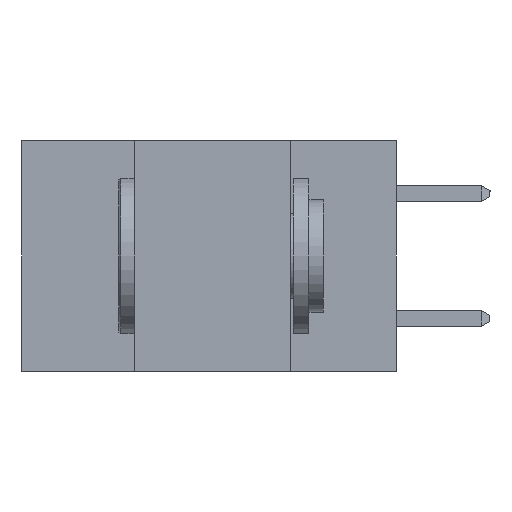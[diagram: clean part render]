
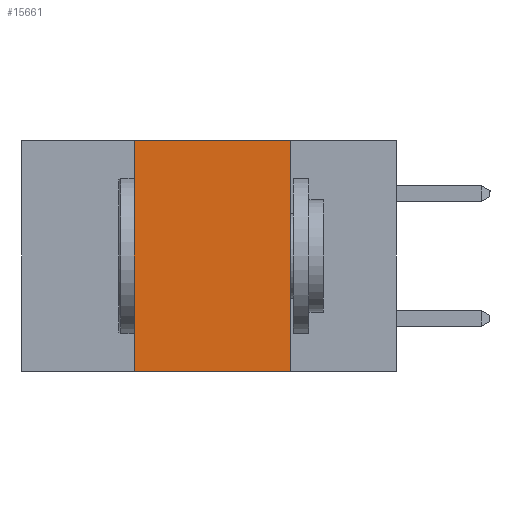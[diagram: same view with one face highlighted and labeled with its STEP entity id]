
A CAD part, left-side view. The second image highlights one B-rep face of the part: STEP entity #15661.
In plain terms, the highlighted planar face has unit normal (-1, 0, 0).
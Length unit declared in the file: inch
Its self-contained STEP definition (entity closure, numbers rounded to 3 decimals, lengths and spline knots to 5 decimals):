
#259 = VECTOR ( 'NONE', #17306, 39.37008 ) ;
#968 = ORIENTED_EDGE ( 'NONE', *, *, #3263, .F. ) ;
#2097 = CARTESIAN_POINT ( 'NONE',  ( 0., 0.6, 0. ) ) ;
#3263 = EDGE_CURVE ( 'NONE', #10058, #10159, #22010, .T. ) ;
#3298 = ORIENTED_EDGE ( 'NONE', *, *, #18414, .F. ) ;
#3435 = VERTEX_POINT ( 'NONE', #24412 ) ;
#3540 = DIRECTION ( 'NONE',  ( 1., 0., 0. ) ) ;
#4045 = CARTESIAN_POINT ( 'NONE',  ( 0., 0.42, -0.37 ) ) ;
#4102 = ORIENTED_EDGE ( 'NONE', *, *, #15124, .T. ) ;
#4536 = LINE ( 'NONE', #12125, #24773 ) ;
#7428 = FACE_OUTER_BOUND ( 'NONE', #17900, .T. ) ;
#8049 = DIRECTION ( 'NONE',  ( 0., 0., 1. ) ) ;
#9212 = LINE ( 'NONE', #15053, #259 ) ;
#10058 = VERTEX_POINT ( 'NONE', #18190 ) ;
#10159 = VERTEX_POINT ( 'NONE', #23187 ) ;
#12125 = CARTESIAN_POINT ( 'NONE',  ( 0., 0.17, -0.37 ) ) ;
#12633 = DIRECTION ( 'NONE',  ( 0., 0., -1. ) ) ;
#13501 = PLANE ( 'NONE',  #24535 ) ;
#13919 = VECTOR ( 'NONE', #8049, 39.37008 ) ;
#15053 = CARTESIAN_POINT ( 'NONE',  ( 0., 0.6, -0.37 ) ) ;
#15124 = EDGE_CURVE ( 'NONE', #10058, #20565, #9212, .T. ) ;
#15511 = CARTESIAN_POINT ( 'NONE',  ( 0., 0.6, 0. ) ) ;
#15661 = ADVANCED_FACE ( 'NONE', ( #7428 ), #13501, .F. ) ;
#17306 = DIRECTION ( 'NONE',  ( 0., -1., 0. ) ) ;
#17900 = EDGE_LOOP ( 'NONE', ( #18639, #3298, #968, #4102 ) ) ;
#18190 = CARTESIAN_POINT ( 'NONE',  ( 0., 0.42, -0.37 ) ) ;
#18414 = EDGE_CURVE ( 'NONE', #10159, #3435, #18718, .T. ) ;
#18639 = ORIENTED_EDGE ( 'NONE', *, *, #18829, .F. ) ;
#18718 = LINE ( 'NONE', #2097, #23909 ) ;
#18829 = EDGE_CURVE ( 'NONE', #3435, #20565, #4536, .T. ) ;
#20242 = CARTESIAN_POINT ( 'NONE',  ( 0., 0.17, -0.37 ) ) ;
#20565 = VERTEX_POINT ( 'NONE', #20242 ) ;
#22010 = LINE ( 'NONE', #4045, #13919 ) ;
#22348 = DIRECTION ( 'NONE',  ( 0., -1., 0. ) ) ;
#23187 = CARTESIAN_POINT ( 'NONE',  ( 0., 0.42, 0. ) ) ;
#23646 = DIRECTION ( 'NONE',  ( 0., 0., -1. ) ) ;
#23909 = VECTOR ( 'NONE', #22348, 39.37008 ) ;
#24412 = CARTESIAN_POINT ( 'NONE',  ( 0., 0.17, 0. ) ) ;
#24535 = AXIS2_PLACEMENT_3D ( 'NONE', #15511, #3540, #23646 ) ;
#24773 = VECTOR ( 'NONE', #12633, 39.37008 ) ;
